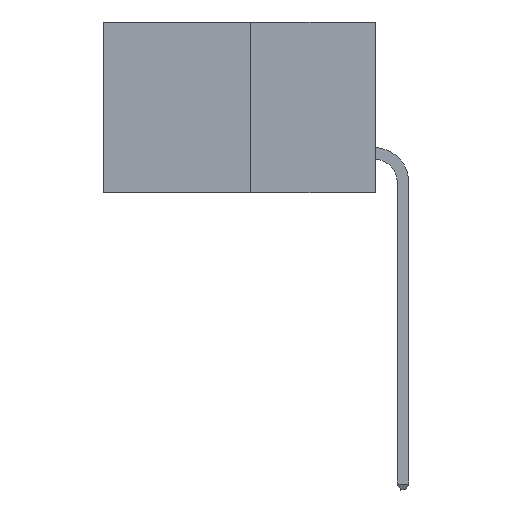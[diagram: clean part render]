
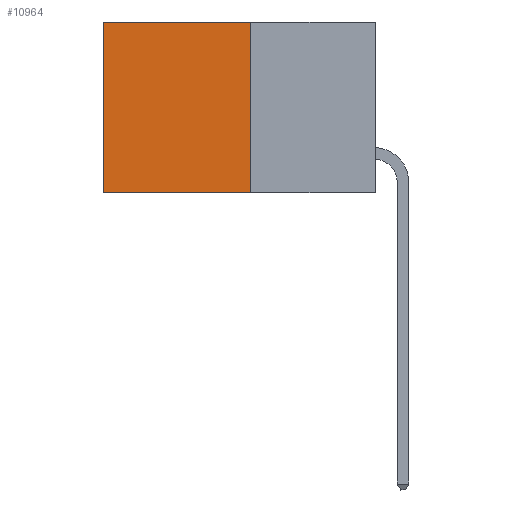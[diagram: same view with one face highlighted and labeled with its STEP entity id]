
A CAD part, left-side view. The second image highlights one B-rep face of the part: STEP entity #10964.
In plain terms, the highlighted planar face has unit normal (-1, 0, 0).
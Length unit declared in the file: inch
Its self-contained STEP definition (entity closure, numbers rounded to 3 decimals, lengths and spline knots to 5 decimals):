
#50 = ORIENTED_EDGE ( 'NONE', *, *, #10838, .F. ) ;
#272 = VERTEX_POINT ( 'NONE', #7168 ) ;
#420 = VERTEX_POINT ( 'NONE', #10751 ) ;
#489 = CARTESIAN_POINT ( 'NONE',  ( 0.277, 0.59, -0.37 ) ) ;
#508 = ORIENTED_EDGE ( 'NONE', *, *, #7445, .T. ) ;
#632 = LINE ( 'NONE', #7115, #9996 ) ;
#1012 = DIRECTION ( 'NONE',  ( 0., 0., -1. ) ) ;
#1091 = CARTESIAN_POINT ( 'NONE',  ( 0.277, 0.27, 0. ) ) ;
#1346 = ORIENTED_EDGE ( 'NONE', *, *, #3953, .T. ) ;
#1420 = FACE_OUTER_BOUND ( 'NONE', #11324, .T. ) ;
#2135 = DIRECTION ( 'NONE',  ( 0., 0., -1. ) ) ;
#2331 = VECTOR ( 'NONE', #11369, 39.37008 ) ;
#2384 = AXIS2_PLACEMENT_3D ( 'NONE', #7716, #5014, #11225 ) ;
#3829 = VERTEX_POINT ( 'NONE', #1091 ) ;
#3953 = EDGE_CURVE ( 'NONE', #3829, #420, #7456, .T. ) ;
#5014 = DIRECTION ( 'NONE',  ( 1., 0., 0. ) ) ;
#5621 = CARTESIAN_POINT ( 'NONE',  ( 0.277, 0.59, -0.37 ) ) ;
#5696 = ORIENTED_EDGE ( 'NONE', *, *, #7229, .F. ) ;
#7115 = CARTESIAN_POINT ( 'NONE',  ( 0.277, 0.27, -0.37 ) ) ;
#7168 = CARTESIAN_POINT ( 'NONE',  ( 0.277, 0.27, -0.37 ) ) ;
#7229 = EDGE_CURVE ( 'NONE', #272, #8743, #632, .T. ) ;
#7445 = EDGE_CURVE ( 'NONE', #420, #8743, #10694, .T. ) ;
#7448 = VECTOR ( 'NONE', #2135, 39.37008 ) ;
#7456 = LINE ( 'NONE', #11408, #2331 ) ;
#7716 = CARTESIAN_POINT ( 'NONE',  ( 0.277, 0.27, -0.37 ) ) ;
#7820 = VECTOR ( 'NONE', #1012, 39.37008 ) ;
#8025 = LINE ( 'NONE', #9317, #7448 ) ;
#8743 = VERTEX_POINT ( 'NONE', #489 ) ;
#9317 = CARTESIAN_POINT ( 'NONE',  ( 0.277, 0.27, -0.37 ) ) ;
#9996 = VECTOR ( 'NONE', #11500, 39.37008 ) ;
#10358 = PLANE ( 'NONE',  #2384 ) ;
#10694 = LINE ( 'NONE', #5621, #7820 ) ;
#10751 = CARTESIAN_POINT ( 'NONE',  ( 0.277, 0.59, 0. ) ) ;
#10838 = EDGE_CURVE ( 'NONE', #3829, #272, #8025, .T. ) ;
#10964 = ADVANCED_FACE ( 'NONE', ( #1420 ), #10358, .F. ) ;
#11225 = DIRECTION ( 'NONE',  ( 0., 0., -1. ) ) ;
#11324 = EDGE_LOOP ( 'NONE', ( #508, #5696, #50, #1346 ) ) ;
#11369 = DIRECTION ( 'NONE',  ( 0., 1., 0. ) ) ;
#11408 = CARTESIAN_POINT ( 'NONE',  ( 0.277, 0.27, 0. ) ) ;
#11500 = DIRECTION ( 'NONE',  ( 0., 1., 0. ) ) ;
